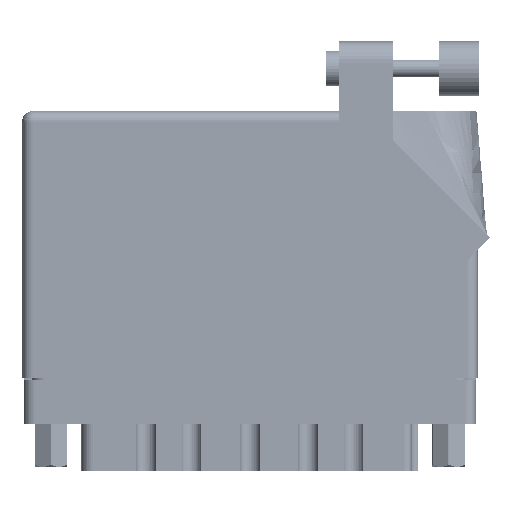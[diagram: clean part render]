
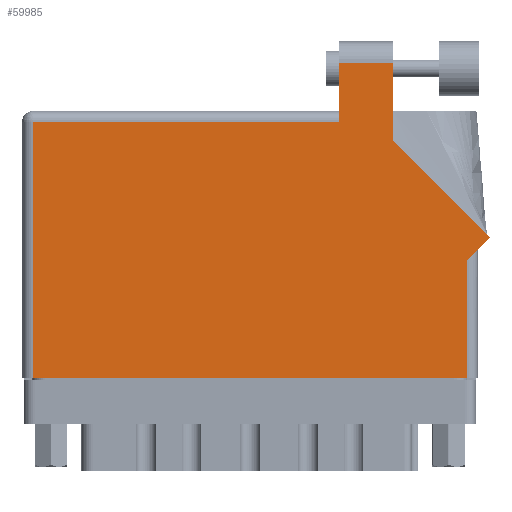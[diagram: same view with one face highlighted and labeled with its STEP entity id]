
A CAD part, front view. The second image highlights one B-rep face of the part: STEP entity #59985.
In plain terms, the highlighted face is planar.
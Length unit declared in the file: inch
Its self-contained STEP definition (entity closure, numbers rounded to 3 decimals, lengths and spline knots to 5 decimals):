
#260 = LINE ( 'NONE', #12882, #4818 ) ;
#2509 = VERTEX_POINT ( 'NONE', #33920 ) ;
#3157 = DIRECTION ( 'NONE',  ( 0., 1., 0. ) ) ;
#3393 = VECTOR ( 'NONE', #15239, 39.37008 ) ;
#3701 = EDGE_CURVE ( 'NONE', #43199, #34723, #49761, .T. ) ;
#4818 = VECTOR ( 'NONE', #3157, 39.37008 ) ;
#5177 = ORIENTED_EDGE ( 'NONE', *, *, #32002, .T. ) ;
#6547 = VERTEX_POINT ( 'NONE', #45937 ) ;
#8130 = DIRECTION ( 'NONE',  ( 0., 0., -1. ) ) ;
#9367 = CARTESIAN_POINT ( 'NONE',  ( 0.062, 0., 0. ) ) ;
#11079 = EDGE_LOOP ( 'NONE', ( #13204, #46820, #47169, #16956, #36647, #29209, #27991, #40378, #5177 ) ) ;
#11831 = VECTOR ( 'NONE', #15417, 39.37008 ) ;
#12039 = EDGE_CURVE ( 'NONE', #14005, #33245, #37441, .T. ) ;
#12882 = CARTESIAN_POINT ( 'NONE',  ( 2.55, 0.737, 0. ) ) ;
#13204 = ORIENTED_EDGE ( 'NONE', *, *, #12039, .T. ) ;
#13582 = DIRECTION ( 'NONE',  ( -1., 0., 0. ) ) ;
#13630 = CARTESIAN_POINT ( 'NONE',  ( 1.819, 1.805, 0. ) ) ;
#14005 = VERTEX_POINT ( 'NONE', #20121 ) ;
#15239 = DIRECTION ( 'NONE',  ( 1., 0., 0. ) ) ;
#15417 = DIRECTION ( 'NONE',  ( 0., 1., 0. ) ) ;
#15527 = CARTESIAN_POINT ( 'NONE',  ( 1.819, 1.468, 0. ) ) ;
#15911 = CARTESIAN_POINT ( 'NONE',  ( 0.062, 0., 0. ) ) ;
#16803 = EDGE_CURVE ( 'NONE', #33245, #43199, #17332, .T. ) ;
#16956 = ORIENTED_EDGE ( 'NONE', *, *, #45626, .T. ) ;
#17332 = LINE ( 'NONE', #22937, #43676 ) ;
#19732 = CARTESIAN_POINT ( 'NONE',  ( 0., 1.468, 0. ) ) ;
#20121 = CARTESIAN_POINT ( 'NONE',  ( 2.126, 1.36442, 0. ) ) ;
#20542 = VECTOR ( 'NONE', #37557, 39.37008 ) ;
#21648 = VECTOR ( 'NONE', #27080, 39.37008 ) ;
#22937 = CARTESIAN_POINT ( 'NONE',  ( 1.819, 1.805, 0. ) ) ;
#24671 = VERTEX_POINT ( 'NONE', #15911 ) ;
#26475 = CARTESIAN_POINT ( 'NONE',  ( 2.612, 0.737, 0. ) ) ;
#27080 = DIRECTION ( 'NONE',  ( 0.707, 0.707, 0. ) ) ;
#27393 = AXIS2_PLACEMENT_3D ( 'NONE', #32134, #8130, #13582 ) ;
#27991 = ORIENTED_EDGE ( 'NONE', *, *, #45013, .T. ) ;
#29209 = ORIENTED_EDGE ( 'NONE', *, *, #60281, .T. ) ;
#30096 = DIRECTION ( 'NONE',  ( 0., -1., 0. ) ) ;
#32002 = EDGE_CURVE ( 'NONE', #6547, #14005, #55985, .T. ) ;
#32134 = CARTESIAN_POINT ( 'NONE',  ( 0., 1.53, 0. ) ) ;
#32392 = EDGE_CURVE ( 'NONE', #2509, #24671, #58967, .T. ) ;
#33245 = VERTEX_POINT ( 'NONE', #38692 ) ;
#33274 = CARTESIAN_POINT ( 'NONE',  ( 2.68271, 0.80771, 0. ) ) ;
#33920 = CARTESIAN_POINT ( 'NONE',  ( 0.062, 1.468, 0. ) ) ;
#34405 = CARTESIAN_POINT ( 'NONE',  ( 0., 0., 0. ) ) ;
#34464 = LINE ( 'NONE', #26475, #21648 ) ;
#34641 = DIRECTION ( 'NONE',  ( -1., 0., 0. ) ) ;
#34723 = VERTEX_POINT ( 'NONE', #15527 ) ;
#34786 = CARTESIAN_POINT ( 'NONE',  ( 2.55, 0.675, 0. ) ) ;
#35619 = LINE ( 'NONE', #19732, #57487 ) ;
#36647 = ORIENTED_EDGE ( 'NONE', *, *, #32392, .T. ) ;
#37441 = LINE ( 'NONE', #54151, #11831 ) ;
#37557 = DIRECTION ( 'NONE',  ( 0., -1., 0. ) ) ;
#37582 = EDGE_CURVE ( 'NONE', #48218, #6547, #34464, .T. ) ;
#38112 = LINE ( 'NONE', #34405, #3393 ) ;
#38692 = CARTESIAN_POINT ( 'NONE',  ( 2.126, 1.805, 0. ) ) ;
#40378 = ORIENTED_EDGE ( 'NONE', *, *, #37582, .T. ) ;
#42092 = DIRECTION ( 'NONE',  ( -1., 0., 0. ) ) ;
#43143 = DIRECTION ( 'NONE',  ( -0.707, 0.707, 0. ) ) ;
#43199 = VERTEX_POINT ( 'NONE', #13630 ) ;
#43676 = VECTOR ( 'NONE', #42092, 39.37008 ) ;
#45013 = EDGE_CURVE ( 'NONE', #50581, #48218, #260, .T. ) ;
#45626 = EDGE_CURVE ( 'NONE', #34723, #2509, #35619, .T. ) ;
#45937 = CARTESIAN_POINT ( 'NONE',  ( 2.68271, 0.80771, 0. ) ) ;
#46433 = FACE_OUTER_BOUND ( 'NONE', #11079, .T. ) ;
#46820 = ORIENTED_EDGE ( 'NONE', *, *, #16803, .T. ) ;
#47169 = ORIENTED_EDGE ( 'NONE', *, *, #3701, .T. ) ;
#48218 = VERTEX_POINT ( 'NONE', #34786 ) ;
#48346 = CARTESIAN_POINT ( 'NONE',  ( 2.55, 0., 0. ) ) ;
#49761 = LINE ( 'NONE', #58712, #53514 ) ;
#49868 = VECTOR ( 'NONE', #43143, 39.37008 ) ;
#50581 = VERTEX_POINT ( 'NONE', #48346 ) ;
#51248 = PLANE ( 'NONE',  #27393 ) ;
#53514 = VECTOR ( 'NONE', #30096, 39.37008 ) ;
#54151 = CARTESIAN_POINT ( 'NONE',  ( 2.126, 1.36442, 0. ) ) ;
#55985 = LINE ( 'NONE', #33274, #49868 ) ;
#57487 = VECTOR ( 'NONE', #34641, 39.37008 ) ;
#58712 = CARTESIAN_POINT ( 'NONE',  ( 1.819, 1.53, 0. ) ) ;
#58967 = LINE ( 'NONE', #9367, #20542 ) ;
#59985 = ADVANCED_FACE ( 'NONE', ( #46433 ), #51248, .F. ) ;
#60281 = EDGE_CURVE ( 'NONE', #24671, #50581, #38112, .T. ) ;
